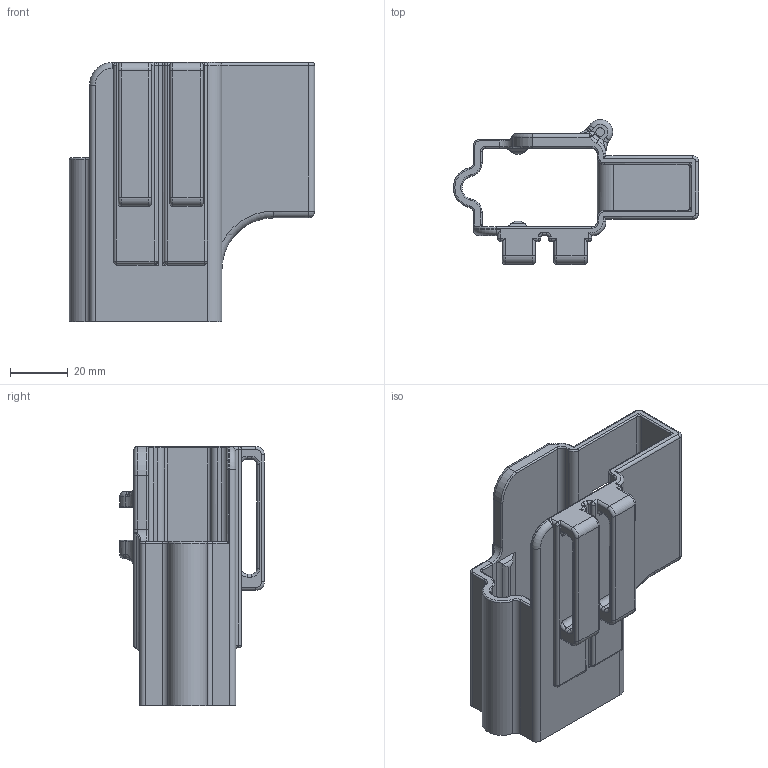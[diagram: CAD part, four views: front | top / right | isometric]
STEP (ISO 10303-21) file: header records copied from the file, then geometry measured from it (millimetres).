
FILE_DESCRIPTION(/* description */ (''),/* implementation_level */ '2;1');
FILE_NAME(/* name */ 'AWCY_43XHOLSTER_FINAL v1.step',/* time_stamp */ '2020-08-17T23:35:52-07:00',/* author */ (''),/* organization */ (''),/* preprocessor_version */ 'ST-DEVELOPER v18.1',/* originating_system */ 'Autodesk Translation Framework v9.3.0.1241',/* authorisation */ '');
FILE_SCHEMA (('AUTOMOTIVE_DESIGN { 1 0 10303 214 3 1 1 }'));
Length unit declared in the file: millimetre
Products named in the file (1): AWCY_43XHOLSTER_FINAL
Bounding box: 85.2 x 50.34 x 90 mm (x, y, z)
Volume: 62972.8 mm3; surface area: 36644.5 mm2
Topology: 1 solids, 1 shells, 771 faces, 2145 edges, 1368 vertices
Faces by surface type: bspline 453, cylinder 149, plane 92, torus 70, sphere 7
Full cylindrical faces by diameter (mm): 3 x2, 9.5 x1
Entity records: 26711 total; most frequent: CARTESIAN_POINT 11109, ORIENTED_EDGE 4268, DIRECTION 2266, EDGE_CURVE 2134, VERTEX_POINT 1368, LINE 828, VECTOR 828, EDGE_LOOP 784
